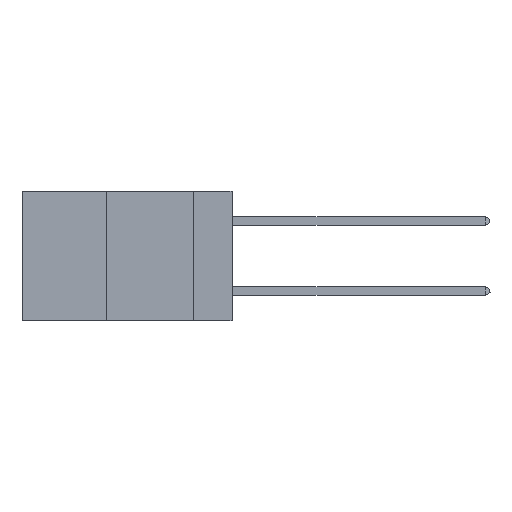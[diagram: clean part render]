
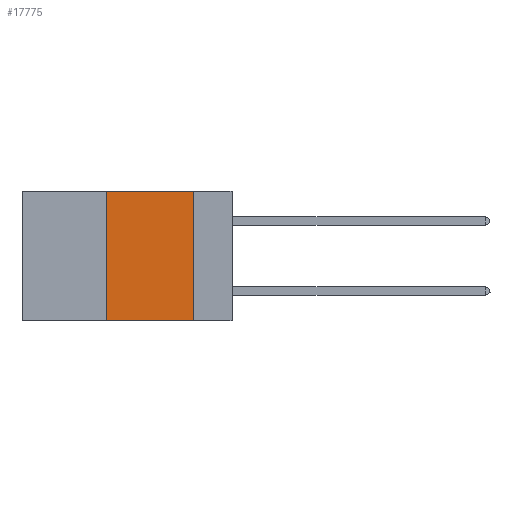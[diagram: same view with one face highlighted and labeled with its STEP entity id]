
A CAD part, left-side view. The second image highlights one B-rep face of the part: STEP entity #17775.
In plain terms, the highlighted planar face has unit normal (-1, 0, 0).
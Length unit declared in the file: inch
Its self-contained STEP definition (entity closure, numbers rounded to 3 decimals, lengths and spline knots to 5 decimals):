
#1145 = DIRECTION ( 'NONE',  ( 0., 0., -1. ) ) ;
#1182 = EDGE_LOOP ( 'NONE', ( #12916, #3581, #14118, #13933 ) ) ;
#1919 = DIRECTION ( 'NONE',  ( 1., 0., 0. ) ) ;
#1924 = VERTEX_POINT ( 'NONE', #12921 ) ;
#2564 = VECTOR ( 'NONE', #9441, 39.37008 ) ;
#2597 = CARTESIAN_POINT ( 'NONE',  ( 0., 0.6, 0. ) ) ;
#3010 = FACE_OUTER_BOUND ( 'NONE', #1182, .T. ) ;
#3386 = LINE ( 'NONE', #2597, #18449 ) ;
#3581 = ORIENTED_EDGE ( 'NONE', *, *, #6465, .F. ) ;
#3657 = DIRECTION ( 'NONE',  ( 0., -1., 0. ) ) ;
#4403 = CARTESIAN_POINT ( 'NONE',  ( 0., 0.11, -0.37 ) ) ;
#4882 = PLANE ( 'NONE',  #9076 ) ;
#5397 = CARTESIAN_POINT ( 'NONE',  ( 0., 0.11, 0. ) ) ;
#6224 = VECTOR ( 'NONE', #1145, 39.37008 ) ;
#6465 = EDGE_CURVE ( 'NONE', #18958, #1924, #3386, .T. ) ;
#6695 = EDGE_CURVE ( 'NONE', #1924, #10657, #13256, .T. ) ;
#7475 = CARTESIAN_POINT ( 'NONE',  ( 0., 0.6, -0.37 ) ) ;
#7822 = CARTESIAN_POINT ( 'NONE',  ( 0., 0.6, 0. ) ) ;
#8000 = LINE ( 'NONE', #17286, #18563 ) ;
#8565 = DIRECTION ( 'NONE',  ( 0., 0., 1. ) ) ;
#9076 = AXIS2_PLACEMENT_3D ( 'NONE', #7822, #1919, #15510 ) ;
#9441 = DIRECTION ( 'NONE',  ( 0., -1., 0. ) ) ;
#10657 = VERTEX_POINT ( 'NONE', #4403 ) ;
#11510 = EDGE_CURVE ( 'NONE', #14761, #10657, #14146, .T. ) ;
#12518 = EDGE_CURVE ( 'NONE', #14761, #18958, #8000, .T. ) ;
#12916 = ORIENTED_EDGE ( 'NONE', *, *, #6695, .F. ) ;
#12921 = CARTESIAN_POINT ( 'NONE',  ( 0., 0.11, 0. ) ) ;
#13256 = LINE ( 'NONE', #5397, #6224 ) ;
#13933 = ORIENTED_EDGE ( 'NONE', *, *, #11510, .T. ) ;
#14118 = ORIENTED_EDGE ( 'NONE', *, *, #12518, .F. ) ;
#14146 = LINE ( 'NONE', #7475, #2564 ) ;
#14761 = VERTEX_POINT ( 'NONE', #17066 ) ;
#15510 = DIRECTION ( 'NONE',  ( 0., 0., -1. ) ) ;
#16071 = CARTESIAN_POINT ( 'NONE',  ( 0., 0.36, 0. ) ) ;
#17066 = CARTESIAN_POINT ( 'NONE',  ( 0., 0.36, -0.37 ) ) ;
#17286 = CARTESIAN_POINT ( 'NONE',  ( 0., 0.36, 0. ) ) ;
#17775 = ADVANCED_FACE ( 'NONE', ( #3010 ), #4882, .F. ) ;
#18449 = VECTOR ( 'NONE', #3657, 39.37008 ) ;
#18563 = VECTOR ( 'NONE', #8565, 39.37008 ) ;
#18958 = VERTEX_POINT ( 'NONE', #16071 ) ;
